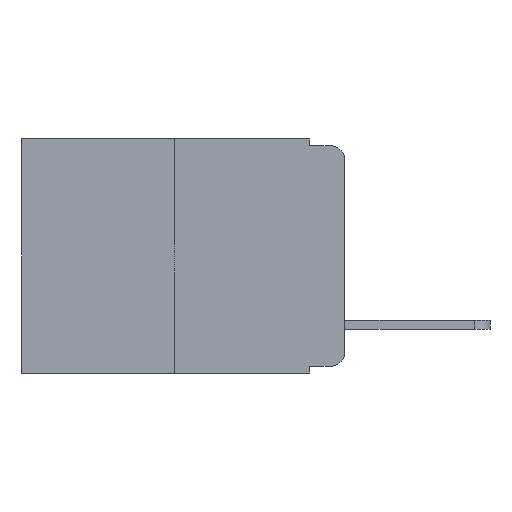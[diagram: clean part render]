
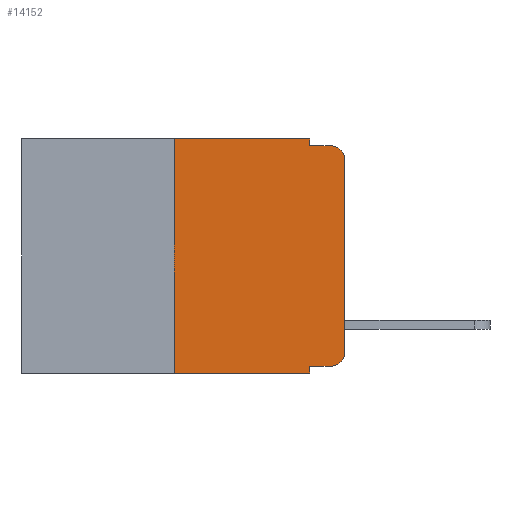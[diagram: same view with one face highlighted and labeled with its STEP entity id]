
A CAD part, left-side view. The second image highlights one B-rep face of the part: STEP entity #14152.
In plain terms, the highlighted planar face has unit normal (-1, 0, 0).
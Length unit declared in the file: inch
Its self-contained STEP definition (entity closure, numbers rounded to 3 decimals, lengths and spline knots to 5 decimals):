
#9 = CARTESIAN_POINT ( 'NONE',  ( 0., 0.051, 0. ) ) ;
#137 = EDGE_LOOP ( 'NONE', ( #18066, #4153, #6646, #958, #1718, #11541, #2050, #19332, #12787, #1246 ) ) ;
#224 = CARTESIAN_POINT ( 'NONE',  ( 0., 0.02, -0.313 ) ) ;
#311 = VECTOR ( 'NONE', #4640, 39.37008 ) ;
#473 = DIRECTION ( 'NONE',  ( 0., -1., 0. ) ) ;
#599 = CARTESIAN_POINT ( 'NONE',  ( 0., 0.051, 0. ) ) ;
#958 = ORIENTED_EDGE ( 'NONE', *, *, #1224, .F. ) ;
#1146 = VERTEX_POINT ( 'NONE', #16176 ) ;
#1150 = VERTEX_POINT ( 'NONE', #16247 ) ;
#1224 = EDGE_CURVE ( 'NONE', #14739, #1150, #7476, .T. ) ;
#1246 = ORIENTED_EDGE ( 'NONE', *, *, #19431, .T. ) ;
#1391 = CARTESIAN_POINT ( 'NONE',  ( 0., 0.02, -0.01 ) ) ;
#1416 = VECTOR ( 'NONE', #17029, 39.37008 ) ;
#1718 = ORIENTED_EDGE ( 'NONE', *, *, #6219, .F. ) ;
#1792 = DIRECTION ( 'NONE',  ( 0., -1., 0. ) ) ;
#2050 = ORIENTED_EDGE ( 'NONE', *, *, #3797, .T. ) ;
#2145 = DIRECTION ( 'NONE',  ( 0., 0., -1. ) ) ;
#2907 = VERTEX_POINT ( 'NONE', #1391 ) ;
#3194 = DIRECTION ( 'NONE',  ( 0., 0., 1. ) ) ;
#3578 = EDGE_CURVE ( 'NONE', #8806, #6480, #4816, .T. ) ;
#3797 = EDGE_CURVE ( 'NONE', #15807, #6480, #18929, .T. ) ;
#4153 = ORIENTED_EDGE ( 'NONE', *, *, #7964, .T. ) ;
#4359 = CARTESIAN_POINT ( 'NONE',  ( 0., 0., -0.313 ) ) ;
#4591 = CARTESIAN_POINT ( 'NONE',  ( 0., 0.02, -0.333 ) ) ;
#4640 = DIRECTION ( 'NONE',  ( 0., 0., -1. ) ) ;
#4654 = DIRECTION ( 'NONE',  ( 0., 0., -1. ) ) ;
#4816 = LINE ( 'NONE', #15077, #311 ) ;
#5247 = DIRECTION ( 'NONE',  ( -1., 0., 0. ) ) ;
#6219 = EDGE_CURVE ( 'NONE', #1146, #14739, #12965, .T. ) ;
#6317 = CARTESIAN_POINT ( 'NONE',  ( 0., 0.25, 0. ) ) ;
#6480 = VERTEX_POINT ( 'NONE', #15105 ) ;
#6646 = ORIENTED_EDGE ( 'NONE', *, *, #17201, .F. ) ;
#6679 = CIRCLE ( 'NONE', #16707, 0.02 ) ;
#7476 = LINE ( 'NONE', #9, #11674 ) ;
#7964 = EDGE_CURVE ( 'NONE', #8370, #2907, #16404, .T. ) ;
#8192 = CARTESIAN_POINT ( 'NONE',  ( 0., 0., -0.03 ) ) ;
#8370 = VERTEX_POINT ( 'NONE', #8192 ) ;
#8426 = CARTESIAN_POINT ( 'NONE',  ( 0., 0.473, 0. ) ) ;
#8536 = CARTESIAN_POINT ( 'NONE',  ( 0., 0.051, -0.01 ) ) ;
#8568 = DIRECTION ( 'NONE',  ( 0., 0., -1. ) ) ;
#8806 = VERTEX_POINT ( 'NONE', #13591 ) ;
#8828 = VERTEX_POINT ( 'NONE', #4591 ) ;
#8891 = CARTESIAN_POINT ( 'NONE',  ( 0., 0.051, -0.333 ) ) ;
#9174 = AXIS2_PLACEMENT_3D ( 'NONE', #11154, #5247, #2145 ) ;
#9236 = VERTEX_POINT ( 'NONE', #4359 ) ;
#9300 = CARTESIAN_POINT ( 'NONE',  ( 0., 0., 0. ) ) ;
#9337 = LINE ( 'NONE', #6317, #13074 ) ;
#9517 = CARTESIAN_POINT ( 'NONE',  ( 0., 0.473, -0.343 ) ) ;
#10540 = DIRECTION ( 'NONE',  ( 0., 0., -1. ) ) ;
#10996 = VECTOR ( 'NONE', #13434, 39.37008 ) ;
#11154 = CARTESIAN_POINT ( 'NONE',  ( 0., 0.02, -0.03 ) ) ;
#11155 = VECTOR ( 'NONE', #473, 39.37008 ) ;
#11541 = ORIENTED_EDGE ( 'NONE', *, *, #17757, .F. ) ;
#11674 = VECTOR ( 'NONE', #10540, 39.37008 ) ;
#12787 = ORIENTED_EDGE ( 'NONE', *, *, #16213, .T. ) ;
#12965 = LINE ( 'NONE', #15433, #18630 ) ;
#13074 = VECTOR ( 'NONE', #3194, 39.37008 ) ;
#13358 = LINE ( 'NONE', #8891, #10996 ) ;
#13434 = DIRECTION ( 'NONE',  ( 0., -1., 0. ) ) ;
#13591 = CARTESIAN_POINT ( 'NONE',  ( 0., 0.051, -0.333 ) ) ;
#13653 = DIRECTION ( 'NONE',  ( -1., 0., 0. ) ) ;
#13978 = CARTESIAN_POINT ( 'NONE',  ( 0., 0.25, -0.343 ) ) ;
#14152 = ADVANCED_FACE ( 'NONE', ( #14501 ), #17380, .F. ) ;
#14237 = VECTOR ( 'NONE', #18965, 39.37008 ) ;
#14375 = AXIS2_PLACEMENT_3D ( 'NONE', #8426, #17318, #8568 ) ;
#14501 = FACE_OUTER_BOUND ( 'NONE', #137, .T. ) ;
#14739 = VERTEX_POINT ( 'NONE', #599 ) ;
#15032 = LINE ( 'NONE', #9300, #1416 ) ;
#15049 = EDGE_CURVE ( 'NONE', #9236, #8370, #15032, .T. ) ;
#15077 = CARTESIAN_POINT ( 'NONE',  ( 0., 0.051, 0. ) ) ;
#15105 = CARTESIAN_POINT ( 'NONE',  ( 0., 0.051, -0.343 ) ) ;
#15433 = CARTESIAN_POINT ( 'NONE',  ( 0., 0.473, 0. ) ) ;
#15807 = VERTEX_POINT ( 'NONE', #13978 ) ;
#16176 = CARTESIAN_POINT ( 'NONE',  ( 0., 0.25, 0. ) ) ;
#16213 = EDGE_CURVE ( 'NONE', #8806, #8828, #13358, .T. ) ;
#16247 = CARTESIAN_POINT ( 'NONE',  ( 0., 0.051, -0.01 ) ) ;
#16404 = CIRCLE ( 'NONE', #9174, 0.02 ) ;
#16707 = AXIS2_PLACEMENT_3D ( 'NONE', #224, #13653, #4654 ) ;
#17029 = DIRECTION ( 'NONE',  ( 0., 0., 1. ) ) ;
#17201 = EDGE_CURVE ( 'NONE', #1150, #2907, #18263, .T. ) ;
#17318 = DIRECTION ( 'NONE',  ( 1., 0., 0. ) ) ;
#17380 = PLANE ( 'NONE',  #14375 ) ;
#17757 = EDGE_CURVE ( 'NONE', #15807, #1146, #9337, .T. ) ;
#18066 = ORIENTED_EDGE ( 'NONE', *, *, #15049, .T. ) ;
#18263 = LINE ( 'NONE', #8536, #14237 ) ;
#18630 = VECTOR ( 'NONE', #1792, 39.37008 ) ;
#18929 = LINE ( 'NONE', #9517, #11155 ) ;
#18965 = DIRECTION ( 'NONE',  ( 0., -1., 0. ) ) ;
#19332 = ORIENTED_EDGE ( 'NONE', *, *, #3578, .F. ) ;
#19431 = EDGE_CURVE ( 'NONE', #8828, #9236, #6679, .T. ) ;
